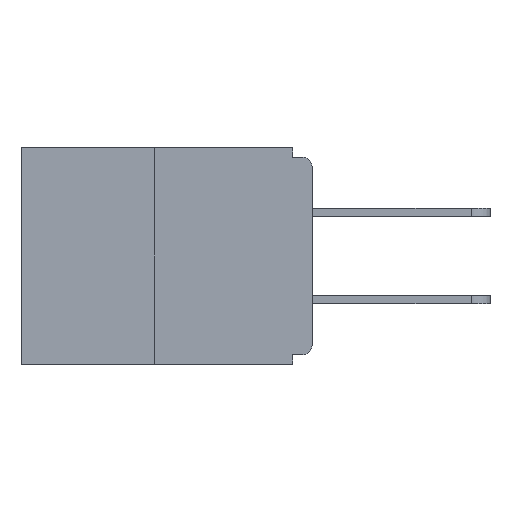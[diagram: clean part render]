
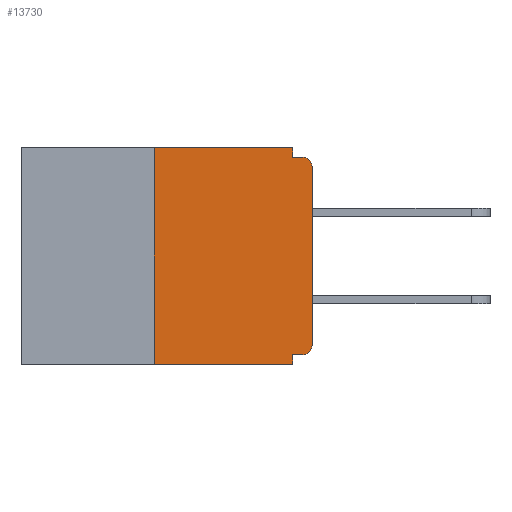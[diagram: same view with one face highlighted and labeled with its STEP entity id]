
A CAD part, left-side view. The second image highlights one B-rep face of the part: STEP entity #13730.
In plain terms, the highlighted planar face has unit normal (-1, 0, 0).
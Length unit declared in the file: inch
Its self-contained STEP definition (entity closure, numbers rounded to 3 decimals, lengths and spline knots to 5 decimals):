
#108 = DIRECTION ( 'NONE',  ( 0., 0., -1. ) ) ;
#120 = LINE ( 'NONE', #18301, #10817 ) ;
#274 = AXIS2_PLACEMENT_3D ( 'NONE', #2192, #310, #2268 ) ;
#310 = DIRECTION ( 'NONE',  ( -1., 0., 0. ) ) ;
#470 = VECTOR ( 'NONE', #12150, 39.37008 ) ;
#656 = VERTEX_POINT ( 'NONE', #21292 ) ;
#1503 = ORIENTED_EDGE ( 'NONE', *, *, #2337, .F. ) ;
#1984 = DIRECTION ( 'NONE',  ( 0., 0., -1. ) ) ;
#2192 = CARTESIAN_POINT ( 'NONE',  ( 0., 0.015, -0.03 ) ) ;
#2268 = DIRECTION ( 'NONE',  ( 0., 0., -1. ) ) ;
#2337 = EDGE_CURVE ( 'NONE', #6040, #4713, #2429, .T. ) ;
#2429 = LINE ( 'NONE', #20459, #5798 ) ;
#2727 = EDGE_CURVE ( 'NONE', #4713, #9709, #21631, .T. ) ;
#2797 = VERTEX_POINT ( 'NONE', #16053 ) ;
#3185 = CARTESIAN_POINT ( 'NONE',  ( 0., 0., -0.313 ) ) ;
#3960 = EDGE_LOOP ( 'NONE', ( #20299, #5165, #17991, #7345, #1503, #10106, #12187, #13267, #7553, #21082 ) ) ;
#4613 = LINE ( 'NONE', #6652, #14525 ) ;
#4713 = VERTEX_POINT ( 'NONE', #5765 ) ;
#4767 = PLANE ( 'NONE',  #19361 ) ;
#4848 = CARTESIAN_POINT ( 'NONE',  ( 0., 0.46, 0. ) ) ;
#4880 = CARTESIAN_POINT ( 'NONE',  ( 0., 0.015, -0.328 ) ) ;
#5165 = ORIENTED_EDGE ( 'NONE', *, *, #11466, .F. ) ;
#5765 = CARTESIAN_POINT ( 'NONE',  ( 0., 0.031, -0.328 ) ) ;
#5798 = VECTOR ( 'NONE', #6052, 39.37008 ) ;
#5886 = CARTESIAN_POINT ( 'NONE',  ( 0., 0.46, -0.343 ) ) ;
#6040 = VERTEX_POINT ( 'NONE', #4880 ) ;
#6052 = DIRECTION ( 'NONE',  ( 0., 1., 0. ) ) ;
#6305 = LINE ( 'NONE', #13528, #15380 ) ;
#6534 = CARTESIAN_POINT ( 'NONE',  ( 0., 0.25, 0. ) ) ;
#6652 = CARTESIAN_POINT ( 'NONE',  ( 0., 0., -0.015 ) ) ;
#7179 = CIRCLE ( 'NONE', #16310, 0.015 ) ;
#7345 = ORIENTED_EDGE ( 'NONE', *, *, #2727, .F. ) ;
#7553 = ORIENTED_EDGE ( 'NONE', *, *, #19883, .F. ) ;
#7586 = DIRECTION ( 'NONE',  ( 1., 0., 0. ) ) ;
#7689 = CARTESIAN_POINT ( 'NONE',  ( 0., 0.25, -0.343 ) ) ;
#7695 = EDGE_CURVE ( 'NONE', #6040, #9815, #7179, .T. ) ;
#8233 = FACE_OUTER_BOUND ( 'NONE', #3960, .T. ) ;
#9691 = VECTOR ( 'NONE', #1984, 39.37008 ) ;
#9709 = VERTEX_POINT ( 'NONE', #16888 ) ;
#9777 = VERTEX_POINT ( 'NONE', #15913 ) ;
#9815 = VERTEX_POINT ( 'NONE', #3185 ) ;
#10106 = ORIENTED_EDGE ( 'NONE', *, *, #7695, .T. ) ;
#10817 = VECTOR ( 'NONE', #11113, 39.37008 ) ;
#11113 = DIRECTION ( 'NONE',  ( 0., 0., 1. ) ) ;
#11125 = LINE ( 'NONE', #19843, #9691 ) ;
#11165 = LINE ( 'NONE', #6534, #470 ) ;
#11194 = CARTESIAN_POINT ( 'NONE',  ( 0., 0.015, -0.313 ) ) ;
#11466 = EDGE_CURVE ( 'NONE', #17908, #16291, #11165, .T. ) ;
#11897 = EDGE_CURVE ( 'NONE', #16291, #21667, #6305, .T. ) ;
#11982 = CARTESIAN_POINT ( 'NONE',  ( 0., 0.031, 0. ) ) ;
#12038 = EDGE_CURVE ( 'NONE', #21667, #2797, #11125, .T. ) ;
#12150 = DIRECTION ( 'NONE',  ( 0., 0., 1. ) ) ;
#12157 = EDGE_CURVE ( 'NONE', #9815, #9777, #120, .T. ) ;
#12187 = ORIENTED_EDGE ( 'NONE', *, *, #12157, .T. ) ;
#13222 = LINE ( 'NONE', #5886, #23400 ) ;
#13267 = ORIENTED_EDGE ( 'NONE', *, *, #17177, .T. ) ;
#13528 = CARTESIAN_POINT ( 'NONE',  ( 0., 0.46, 0. ) ) ;
#13730 = ADVANCED_FACE ( 'NONE', ( #8233 ), #4767, .F. ) ;
#14525 = VECTOR ( 'NONE', #15690, 39.37008 ) ;
#15380 = VECTOR ( 'NONE', #22631, 39.37008 ) ;
#15383 = CARTESIAN_POINT ( 'NONE',  ( 0., 0.031, -0.343 ) ) ;
#15401 = VECTOR ( 'NONE', #16433, 39.37008 ) ;
#15690 = DIRECTION ( 'NONE',  ( 0., -1., 0. ) ) ;
#15913 = CARTESIAN_POINT ( 'NONE',  ( 0., 0., -0.03 ) ) ;
#16053 = CARTESIAN_POINT ( 'NONE',  ( 0., 0.031, -0.015 ) ) ;
#16229 = EDGE_CURVE ( 'NONE', #17908, #9709, #13222, .T. ) ;
#16291 = VERTEX_POINT ( 'NONE', #16734 ) ;
#16310 = AXIS2_PLACEMENT_3D ( 'NONE', #11194, #21956, #22121 ) ;
#16433 = DIRECTION ( 'NONE',  ( 0., 0., -1. ) ) ;
#16734 = CARTESIAN_POINT ( 'NONE',  ( 0., 0.25, 0. ) ) ;
#16888 = CARTESIAN_POINT ( 'NONE',  ( 0., 0.031, -0.343 ) ) ;
#17177 = EDGE_CURVE ( 'NONE', #9777, #656, #21127, .T. ) ;
#17908 = VERTEX_POINT ( 'NONE', #7689 ) ;
#17991 = ORIENTED_EDGE ( 'NONE', *, *, #16229, .T. ) ;
#18301 = CARTESIAN_POINT ( 'NONE',  ( 0., 0., 0. ) ) ;
#18741 = DIRECTION ( 'NONE',  ( 0., -1., 0. ) ) ;
#19361 = AXIS2_PLACEMENT_3D ( 'NONE', #4848, #7586, #108 ) ;
#19843 = CARTESIAN_POINT ( 'NONE',  ( 0., 0.031, 0. ) ) ;
#19883 = EDGE_CURVE ( 'NONE', #2797, #656, #4613, .T. ) ;
#20299 = ORIENTED_EDGE ( 'NONE', *, *, #11897, .F. ) ;
#20459 = CARTESIAN_POINT ( 'NONE',  ( 0., 0., -0.328 ) ) ;
#21082 = ORIENTED_EDGE ( 'NONE', *, *, #12038, .F. ) ;
#21127 = CIRCLE ( 'NONE', #274, 0.015 ) ;
#21292 = CARTESIAN_POINT ( 'NONE',  ( 0., 0.015, -0.015 ) ) ;
#21631 = LINE ( 'NONE', #15383, #15401 ) ;
#21667 = VERTEX_POINT ( 'NONE', #11982 ) ;
#21956 = DIRECTION ( 'NONE',  ( -1., 0., 0. ) ) ;
#22121 = DIRECTION ( 'NONE',  ( 0., 0., -1. ) ) ;
#22631 = DIRECTION ( 'NONE',  ( 0., -1., 0. ) ) ;
#23400 = VECTOR ( 'NONE', #18741, 39.37008 ) ;
